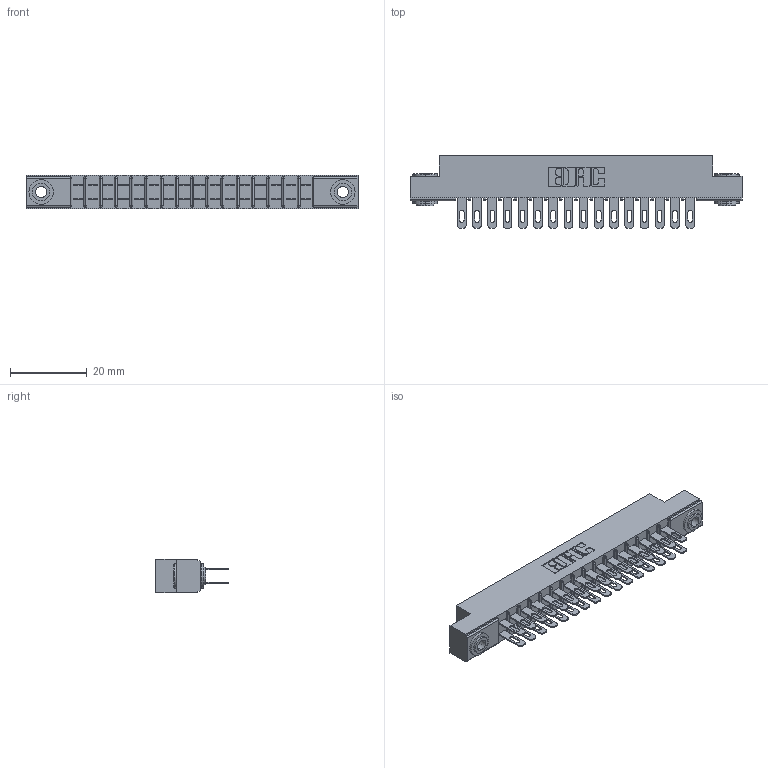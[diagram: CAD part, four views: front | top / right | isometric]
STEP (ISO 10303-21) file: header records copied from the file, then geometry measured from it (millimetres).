
FILE_DESCRIPTION (( 'STEP AP203' ), '1' );
FILE_NAME ('355-032-500-203.STEP', '2019-09-11T07:35:13', ( '' ), ( '' ), 'SwSTEP 2.0', 'SolidWorks 2016', '' );
FILE_SCHEMA (( 'CONFIG_CONTROL_DESIGN' ));
Length unit declared in the file: inch
Products named in the file (4): 345-250-002_345-250-002-102; 355-032-500-203; 305-290-001_500; 305 Part_.156 Dia
Assembly tree (35 placements, depth 2):
  355-032-500-203
    305 Part_.156 Dia
    305-290-001_500  x32
    345-250-002_345-250-002-102  x2
Bounding box: 86.41 x 18.85 x 8.71 mm (x, y, z)
Volume: 5524.7 mm3; surface area: 10902.1 mm2
Topology: 35 solids, 35 shells, 1768 faces, 5020 edges, 3256 vertices
Faces by surface type: plane 988, cylinder 708, sphere 64, cone 8
Entity records: 21576 total; most frequent: CARTESIAN_POINT 3551, ORIENTED_EDGE 3512, DIRECTION 3474, EDGE_CURVE 1756, LINE 1380, VECTOR 1380, VERTEX_POINT 1124, AXIS2_PLACEMENT_3D 1047
